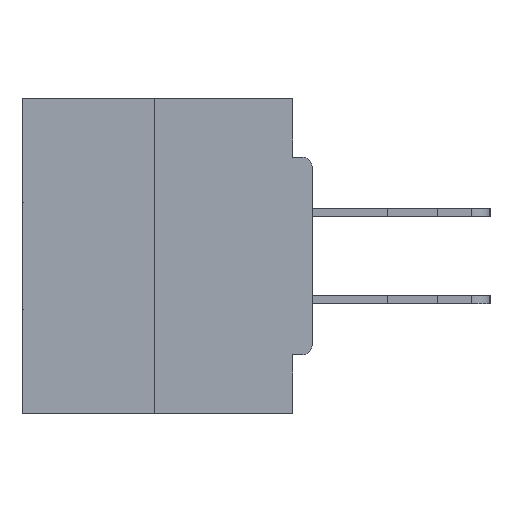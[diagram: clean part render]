
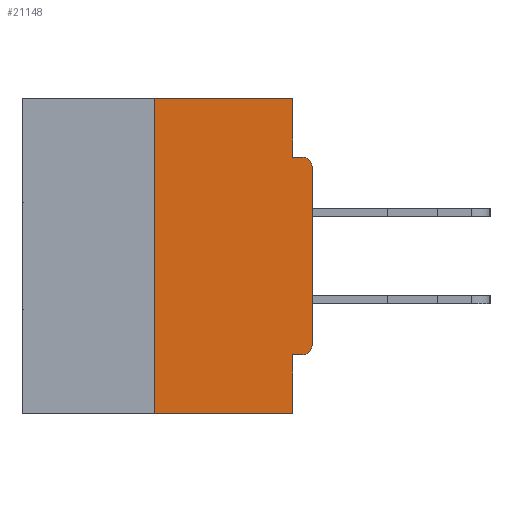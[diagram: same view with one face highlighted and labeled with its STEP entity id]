
A CAD part, left-side view. The second image highlights one B-rep face of the part: STEP entity #21148.
In plain terms, the highlighted planar face has unit normal (-1, 0, 0).
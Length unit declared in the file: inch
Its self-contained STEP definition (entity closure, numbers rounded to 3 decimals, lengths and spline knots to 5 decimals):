
#460 = VERTEX_POINT ( 'NONE', #2924 ) ;
#667 = VECTOR ( 'NONE', #33892, 39.37008 ) ;
#842 = VECTOR ( 'NONE', #20309, 39.37008 ) ;
#1342 = DIRECTION ( 'NONE',  ( 0., -1., 0. ) ) ;
#1692 = VERTEX_POINT ( 'NONE', #10401 ) ;
#1750 = AXIS2_PLACEMENT_3D ( 'NONE', #27031, #12133, #27229 ) ;
#1991 = DIRECTION ( 'NONE',  ( 0., -1., 0. ) ) ;
#2367 = LINE ( 'NONE', #19638, #18619 ) ;
#2379 = CARTESIAN_POINT ( 'NONE',  ( 0., 0.015, -0.4065 ) ) ;
#2481 = DIRECTION ( 'NONE',  ( 0., 0., -1. ) ) ;
#2706 = VECTOR ( 'NONE', #1342, 39.37008 ) ;
#2924 = CARTESIAN_POINT ( 'NONE',  ( 0., 0., -0.1085 ) ) ;
#3861 = EDGE_CURVE ( 'NONE', #17601, #24856, #2367, .T. ) ;
#4117 = CARTESIAN_POINT ( 'NONE',  ( 0., 0.46, -0.5 ) ) ;
#4379 = VERTEX_POINT ( 'NONE', #17776 ) ;
#4758 = CARTESIAN_POINT ( 'NONE',  ( 0., 0., -0.0935 ) ) ;
#5450 = CIRCLE ( 'NONE', #15572, 0.015 ) ;
#6406 = CARTESIAN_POINT ( 'NONE',  ( 0., 0.031, -0.5 ) ) ;
#6547 = EDGE_CURVE ( 'NONE', #12844, #19053, #38903, .T. ) ;
#6847 = EDGE_LOOP ( 'NONE', ( #26934, #10889, #26144, #24114, #21053, #23297, #16322, #8209, #15326, #29923 ) ) ;
#7500 = CARTESIAN_POINT ( 'NONE',  ( 0., 0.031, -0.5 ) ) ;
#8197 = VERTEX_POINT ( 'NONE', #37728 ) ;
#8209 = ORIENTED_EDGE ( 'NONE', *, *, #28052, .T. ) ;
#9203 = CARTESIAN_POINT ( 'NONE',  ( 0., 0.015, -0.1085 ) ) ;
#9755 = CARTESIAN_POINT ( 'NONE',  ( 0., 0., -0.3915 ) ) ;
#10401 = CARTESIAN_POINT ( 'NONE',  ( 0., 0.25, -0.5 ) ) ;
#10889 = ORIENTED_EDGE ( 'NONE', *, *, #19482, .F. ) ;
#11948 = LINE ( 'NONE', #17704, #20102 ) ;
#12133 = DIRECTION ( 'NONE',  ( 1., 0., 0. ) ) ;
#12844 = VERTEX_POINT ( 'NONE', #14143 ) ;
#13474 = EDGE_CURVE ( 'NONE', #17601, #28580, #5450, .T. ) ;
#13611 = LINE ( 'NONE', #4117, #2706 ) ;
#14143 = CARTESIAN_POINT ( 'NONE',  ( 0., 0.031, 0. ) ) ;
#14543 = CARTESIAN_POINT ( 'NONE',  ( 0., 0., 0. ) ) ;
#15209 = VERTEX_POINT ( 'NONE', #6406 ) ;
#15227 = AXIS2_PLACEMENT_3D ( 'NONE', #9203, #21318, #2481 ) ;
#15326 = ORIENTED_EDGE ( 'NONE', *, *, #38431, .F. ) ;
#15572 = AXIS2_PLACEMENT_3D ( 'NONE', #28348, #22377, #34466 ) ;
#16322 = ORIENTED_EDGE ( 'NONE', *, *, #30303, .T. ) ;
#16804 = EDGE_CURVE ( 'NONE', #24856, #15209, #34474, .T. ) ;
#17125 = CIRCLE ( 'NONE', #15227, 0.015 ) ;
#17293 = CARTESIAN_POINT ( 'NONE',  ( 0., 0.031, -0.0935 ) ) ;
#17601 = VERTEX_POINT ( 'NONE', #2379 ) ;
#17704 = CARTESIAN_POINT ( 'NONE',  ( 0., 0.46, 0. ) ) ;
#17776 = CARTESIAN_POINT ( 'NONE',  ( 0., 0.015, -0.0935 ) ) ;
#17922 = CARTESIAN_POINT ( 'NONE',  ( 0., 0.25, 0. ) ) ;
#18619 = VECTOR ( 'NONE', #38463, 39.37008 ) ;
#19053 = VERTEX_POINT ( 'NONE', #17293 ) ;
#19482 = EDGE_CURVE ( 'NONE', #1692, #8197, #21896, .T. ) ;
#19638 = CARTESIAN_POINT ( 'NONE',  ( 0., 0., -0.4065 ) ) ;
#20102 = VECTOR ( 'NONE', #38930, 39.37008 ) ;
#20309 = DIRECTION ( 'NONE',  ( 0., 0., 1. ) ) ;
#21053 = ORIENTED_EDGE ( 'NONE', *, *, #3861, .F. ) ;
#21148 = ADVANCED_FACE ( 'NONE', ( #33754 ), #33158, .F. ) ;
#21318 = DIRECTION ( 'NONE',  ( -1., 0., 0. ) ) ;
#21896 = LINE ( 'NONE', #17922, #37084 ) ;
#22377 = DIRECTION ( 'NONE',  ( -1., 0., 0. ) ) ;
#23297 = ORIENTED_EDGE ( 'NONE', *, *, #13474, .T. ) ;
#23830 = DIRECTION ( 'NONE',  ( 0., 0., -1. ) ) ;
#24114 = ORIENTED_EDGE ( 'NONE', *, *, #16804, .F. ) ;
#24856 = VERTEX_POINT ( 'NONE', #34827 ) ;
#25681 = EDGE_CURVE ( 'NONE', #8197, #12844, #11948, .T. ) ;
#26144 = ORIENTED_EDGE ( 'NONE', *, *, #34734, .T. ) ;
#26473 = LINE ( 'NONE', #14543, #842 ) ;
#26934 = ORIENTED_EDGE ( 'NONE', *, *, #25681, .F. ) ;
#27031 = CARTESIAN_POINT ( 'NONE',  ( 0., 0.46, 0. ) ) ;
#27229 = DIRECTION ( 'NONE',  ( 0., 0., -1. ) ) ;
#28052 = EDGE_CURVE ( 'NONE', #460, #4379, #17125, .T. ) ;
#28348 = CARTESIAN_POINT ( 'NONE',  ( 0., 0.015, -0.3915 ) ) ;
#28580 = VERTEX_POINT ( 'NONE', #9755 ) ;
#29461 = VECTOR ( 'NONE', #1991, 39.37008 ) ;
#29592 = CARTESIAN_POINT ( 'NONE',  ( 0., 0.031, 0. ) ) ;
#29923 = ORIENTED_EDGE ( 'NONE', *, *, #6547, .F. ) ;
#30303 = EDGE_CURVE ( 'NONE', #28580, #460, #26473, .T. ) ;
#32697 = VECTOR ( 'NONE', #23830, 39.37008 ) ;
#33158 = PLANE ( 'NONE',  #1750 ) ;
#33754 = FACE_OUTER_BOUND ( 'NONE', #6847, .T. ) ;
#33892 = DIRECTION ( 'NONE',  ( 0., 0., -1. ) ) ;
#34466 = DIRECTION ( 'NONE',  ( 0., 0., -1. ) ) ;
#34474 = LINE ( 'NONE', #7500, #667 ) ;
#34734 = EDGE_CURVE ( 'NONE', #1692, #15209, #13611, .T. ) ;
#34827 = CARTESIAN_POINT ( 'NONE',  ( 0., 0.031, -0.4065 ) ) ;
#36182 = DIRECTION ( 'NONE',  ( 0., 0., 1. ) ) ;
#37084 = VECTOR ( 'NONE', #36182, 39.37008 ) ;
#37728 = CARTESIAN_POINT ( 'NONE',  ( 0., 0.25, 0. ) ) ;
#38273 = LINE ( 'NONE', #4758, #29461 ) ;
#38431 = EDGE_CURVE ( 'NONE', #19053, #4379, #38273, .T. ) ;
#38463 = DIRECTION ( 'NONE',  ( 0., 1., 0. ) ) ;
#38903 = LINE ( 'NONE', #29592, #32697 ) ;
#38930 = DIRECTION ( 'NONE',  ( 0., -1., 0. ) ) ;
